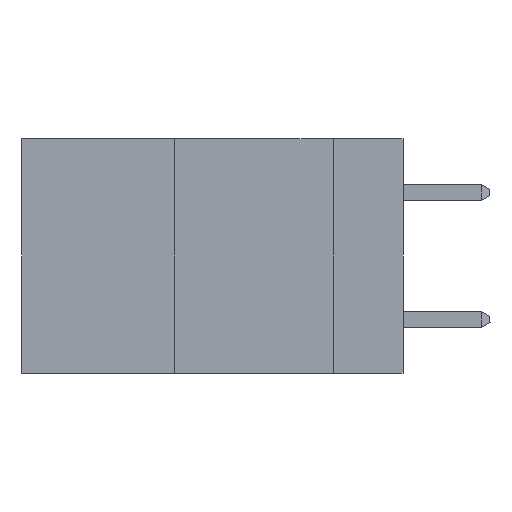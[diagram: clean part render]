
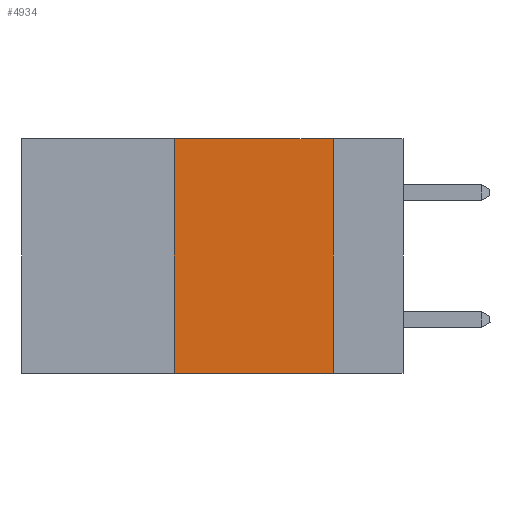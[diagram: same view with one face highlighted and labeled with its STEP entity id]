
A CAD part, left-side view. The second image highlights one B-rep face of the part: STEP entity #4934.
In plain terms, the highlighted planar face has unit normal (-1, 0, 0).
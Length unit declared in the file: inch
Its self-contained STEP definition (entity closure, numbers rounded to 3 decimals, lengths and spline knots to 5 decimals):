
#1316 = VECTOR ( 'NONE', #18572, 39.37008 ) ;
#1766 = AXIS2_PLACEMENT_3D ( 'NONE', #29859, #28070, #19467 ) ;
#2093 = DIRECTION ( 'NONE',  ( 0., 0., -1. ) ) ;
#3423 = CARTESIAN_POINT ( 'NONE',  ( 0., 0.6, -0.37 ) ) ;
#4336 = ORIENTED_EDGE ( 'NONE', *, *, #25205, .F. ) ;
#4934 = ADVANCED_FACE ( 'NONE', ( #7126 ), #16860, .F. ) ;
#5049 = ORIENTED_EDGE ( 'NONE', *, *, #5639, .F. ) ;
#5639 = EDGE_CURVE ( 'NONE', #30039, #11676, #27131, .T. ) ;
#5812 = CARTESIAN_POINT ( 'NONE',  ( 0., 0.11, -0.37 ) ) ;
#7126 = FACE_OUTER_BOUND ( 'NONE', #22007, .T. ) ;
#7986 = CARTESIAN_POINT ( 'NONE',  ( 0., 0.11, 0. ) ) ;
#8020 = CARTESIAN_POINT ( 'NONE',  ( 0., 0.6, 0. ) ) ;
#9429 = ORIENTED_EDGE ( 'NONE', *, *, #27596, .T. ) ;
#10950 = VECTOR ( 'NONE', #24365, 39.37008 ) ;
#11560 = LINE ( 'NONE', #3423, #20783 ) ;
#11676 = VERTEX_POINT ( 'NONE', #11789 ) ;
#11789 = CARTESIAN_POINT ( 'NONE',  ( 0., 0.36, 0. ) ) ;
#13177 = EDGE_CURVE ( 'NONE', #27409, #30327, #21145, .T. ) ;
#16860 = PLANE ( 'NONE',  #1766 ) ;
#18572 = DIRECTION ( 'NONE',  ( 0., -1., 0. ) ) ;
#19467 = DIRECTION ( 'NONE',  ( 0., 0., -1. ) ) ;
#20783 = VECTOR ( 'NONE', #26967, 39.37008 ) ;
#20881 = ORIENTED_EDGE ( 'NONE', *, *, #13177, .F. ) ;
#21145 = LINE ( 'NONE', #7986, #31054 ) ;
#22007 = EDGE_LOOP ( 'NONE', ( #20881, #4336, #5049, #9429 ) ) ;
#23134 = CARTESIAN_POINT ( 'NONE',  ( 0., 0.36, -0.37 ) ) ;
#24365 = DIRECTION ( 'NONE',  ( 0., 0., 1. ) ) ;
#25205 = EDGE_CURVE ( 'NONE', #11676, #27409, #31750, .T. ) ;
#25433 = CARTESIAN_POINT ( 'NONE',  ( 0., 0.11, 0. ) ) ;
#26967 = DIRECTION ( 'NONE',  ( 0., -1., 0. ) ) ;
#27131 = LINE ( 'NONE', #29559, #10950 ) ;
#27409 = VERTEX_POINT ( 'NONE', #25433 ) ;
#27596 = EDGE_CURVE ( 'NONE', #30039, #30327, #11560, .T. ) ;
#28070 = DIRECTION ( 'NONE',  ( 1., 0., 0. ) ) ;
#29559 = CARTESIAN_POINT ( 'NONE',  ( 0., 0.36, 0. ) ) ;
#29859 = CARTESIAN_POINT ( 'NONE',  ( 0., 0.6, 0. ) ) ;
#30039 = VERTEX_POINT ( 'NONE', #23134 ) ;
#30327 = VERTEX_POINT ( 'NONE', #5812 ) ;
#31054 = VECTOR ( 'NONE', #2093, 39.37008 ) ;
#31750 = LINE ( 'NONE', #8020, #1316 ) ;
